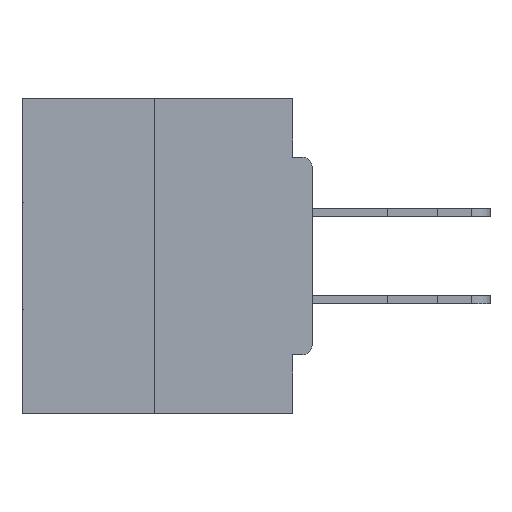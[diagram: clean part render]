
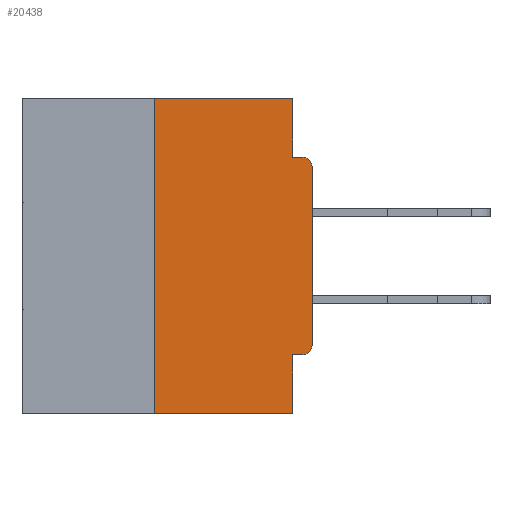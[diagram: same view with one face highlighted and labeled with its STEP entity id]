
A CAD part, left-side view. The second image highlights one B-rep face of the part: STEP entity #20438.
In plain terms, the highlighted planar face has unit normal (-1, 0, 0).
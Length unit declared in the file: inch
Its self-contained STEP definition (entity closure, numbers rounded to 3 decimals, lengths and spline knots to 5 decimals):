
#2 = VERTEX_POINT ( 'NONE', #33842 ) ;
#215 = VECTOR ( 'NONE', #5214, 39.37008 ) ;
#308 = CARTESIAN_POINT ( 'NONE',  ( 0., 0.015, -0.3915 ) ) ;
#803 = CARTESIAN_POINT ( 'NONE',  ( 0., 0.031, -0.5 ) ) ;
#864 = VERTEX_POINT ( 'NONE', #24918 ) ;
#1313 = EDGE_CURVE ( 'NONE', #37869, #864, #27693, .T. ) ;
#1557 = CARTESIAN_POINT ( 'NONE',  ( 0., 0.015, -0.4065 ) ) ;
#1784 = LINE ( 'NONE', #24470, #17371 ) ;
#2678 = ORIENTED_EDGE ( 'NONE', *, *, #26052, .T. ) ;
#2728 = VECTOR ( 'NONE', #30642, 39.37008 ) ;
#3273 = DIRECTION ( 'NONE',  ( 0., 0., 1. ) ) ;
#4671 = ORIENTED_EDGE ( 'NONE', *, *, #27276, .F. ) ;
#4835 = CIRCLE ( 'NONE', #23643, 0.015 ) ;
#5214 = DIRECTION ( 'NONE',  ( 0., 0., -1. ) ) ;
#5887 = CARTESIAN_POINT ( 'NONE',  ( 0., 0.25, 0. ) ) ;
#6461 = CARTESIAN_POINT ( 'NONE',  ( 0., 0.015, -0.1085 ) ) ;
#6607 = CARTESIAN_POINT ( 'NONE',  ( 0., 0., 0. ) ) ;
#7156 = DIRECTION ( 'NONE',  ( 0., -1., 0. ) ) ;
#7268 = VERTEX_POINT ( 'NONE', #8518 ) ;
#8225 = AXIS2_PLACEMENT_3D ( 'NONE', #6461, #31033, #21551 ) ;
#8518 = CARTESIAN_POINT ( 'NONE',  ( 0., 0.25, -0.5 ) ) ;
#8785 = CARTESIAN_POINT ( 'NONE',  ( 0., 0.031, -0.0935 ) ) ;
#9221 = CARTESIAN_POINT ( 'NONE',  ( 0., 0.031, -0.4065 ) ) ;
#9676 = DIRECTION ( 'NONE',  ( 0., 0., -1. ) ) ;
#10077 = DIRECTION ( 'NONE',  ( 0., -1., 0. ) ) ;
#10229 = VECTOR ( 'NONE', #9676, 39.37008 ) ;
#11316 = EDGE_LOOP ( 'NONE', ( #35311, #30005, #2678, #4671, #26817, #12526, #11748, #37493, #36827, #17884 ) ) ;
#11748 = ORIENTED_EDGE ( 'NONE', *, *, #1313, .T. ) ;
#12216 = DIRECTION ( 'NONE',  ( -1., 0., 0. ) ) ;
#12526 = ORIENTED_EDGE ( 'NONE', *, *, #32339, .T. ) ;
#12895 = DIRECTION ( 'NONE',  ( 0., -1., 0. ) ) ;
#13193 = CARTESIAN_POINT ( 'NONE',  ( 0., 0.46, -0.5 ) ) ;
#13472 = LINE ( 'NONE', #38195, #215 ) ;
#13923 = VECTOR ( 'NONE', #20188, 39.37008 ) ;
#14433 = VECTOR ( 'NONE', #7156, 39.37008 ) ;
#15664 = EDGE_CURVE ( 'NONE', #37945, #22243, #13472, .T. ) ;
#16493 = CARTESIAN_POINT ( 'NONE',  ( 0., 0.46, 0. ) ) ;
#16593 = VECTOR ( 'NONE', #10077, 39.37008 ) ;
#16669 = VERTEX_POINT ( 'NONE', #1557 ) ;
#17371 = VECTOR ( 'NONE', #3273, 39.37008 ) ;
#17884 = ORIENTED_EDGE ( 'NONE', *, *, #15664, .F. ) ;
#19068 = EDGE_CURVE ( 'NONE', #22243, #33959, #30124, .T. ) ;
#19276 = CARTESIAN_POINT ( 'NONE',  ( 0., 0.46, 0. ) ) ;
#19526 = PLANE ( 'NONE',  #26320 ) ;
#20188 = DIRECTION ( 'NONE',  ( 0., 1., 0. ) ) ;
#20337 = LINE ( 'NONE', #16493, #16593 ) ;
#20438 = ADVANCED_FACE ( 'NONE', ( #37994 ), #19526, .F. ) ;
#21070 = LINE ( 'NONE', #803, #10229 ) ;
#21120 = EDGE_CURVE ( 'NONE', #864, #33959, #29020, .T. ) ;
#21551 = DIRECTION ( 'NONE',  ( 0., 0., -1. ) ) ;
#21657 = DIRECTION ( 'NONE',  ( 0., 0., -1. ) ) ;
#22243 = VERTEX_POINT ( 'NONE', #8785 ) ;
#23643 = AXIS2_PLACEMENT_3D ( 'NONE', #308, #12216, #21657 ) ;
#24470 = CARTESIAN_POINT ( 'NONE',  ( 0., 0.25, 0. ) ) ;
#24775 = LINE ( 'NONE', #13193, #14433 ) ;
#24918 = CARTESIAN_POINT ( 'NONE',  ( 0., 0., -0.1085 ) ) ;
#25892 = VECTOR ( 'NONE', #12895, 39.37008 ) ;
#26052 = EDGE_CURVE ( 'NONE', #7268, #2, #24775, .T. ) ;
#26320 = AXIS2_PLACEMENT_3D ( 'NONE', #19276, #31869, #29239 ) ;
#26376 = CARTESIAN_POINT ( 'NONE',  ( 0., 0., -0.3915 ) ) ;
#26677 = VERTEX_POINT ( 'NONE', #9221 ) ;
#26817 = ORIENTED_EDGE ( 'NONE', *, *, #33879, .F. ) ;
#27155 = CARTESIAN_POINT ( 'NONE',  ( 0., 0.015, -0.0935 ) ) ;
#27276 = EDGE_CURVE ( 'NONE', #26677, #2, #21070, .T. ) ;
#27337 = EDGE_CURVE ( 'NONE', #36629, #37945, #20337, .T. ) ;
#27693 = LINE ( 'NONE', #6607, #2728 ) ;
#29020 = CIRCLE ( 'NONE', #8225, 0.015 ) ;
#29239 = DIRECTION ( 'NONE',  ( 0., 0., -1. ) ) ;
#29474 = EDGE_CURVE ( 'NONE', #7268, #36629, #1784, .T. ) ;
#30005 = ORIENTED_EDGE ( 'NONE', *, *, #29474, .F. ) ;
#30124 = LINE ( 'NONE', #33228, #25892 ) ;
#30642 = DIRECTION ( 'NONE',  ( 0., 0., 1. ) ) ;
#30887 = LINE ( 'NONE', #35538, #13923 ) ;
#31033 = DIRECTION ( 'NONE',  ( -1., 0., 0. ) ) ;
#31869 = DIRECTION ( 'NONE',  ( 1., 0., 0. ) ) ;
#32339 = EDGE_CURVE ( 'NONE', #16669, #37869, #4835, .T. ) ;
#33228 = CARTESIAN_POINT ( 'NONE',  ( 0., 0., -0.0935 ) ) ;
#33842 = CARTESIAN_POINT ( 'NONE',  ( 0., 0.031, -0.5 ) ) ;
#33879 = EDGE_CURVE ( 'NONE', #16669, #26677, #30887, .T. ) ;
#33959 = VERTEX_POINT ( 'NONE', #27155 ) ;
#35311 = ORIENTED_EDGE ( 'NONE', *, *, #27337, .F. ) ;
#35538 = CARTESIAN_POINT ( 'NONE',  ( 0., 0., -0.4065 ) ) ;
#36629 = VERTEX_POINT ( 'NONE', #5887 ) ;
#36827 = ORIENTED_EDGE ( 'NONE', *, *, #19068, .F. ) ;
#37493 = ORIENTED_EDGE ( 'NONE', *, *, #21120, .T. ) ;
#37869 = VERTEX_POINT ( 'NONE', #26376 ) ;
#37945 = VERTEX_POINT ( 'NONE', #38978 ) ;
#37994 = FACE_OUTER_BOUND ( 'NONE', #11316, .T. ) ;
#38195 = CARTESIAN_POINT ( 'NONE',  ( 0., 0.031, 0. ) ) ;
#38978 = CARTESIAN_POINT ( 'NONE',  ( 0., 0.031, 0. ) ) ;
